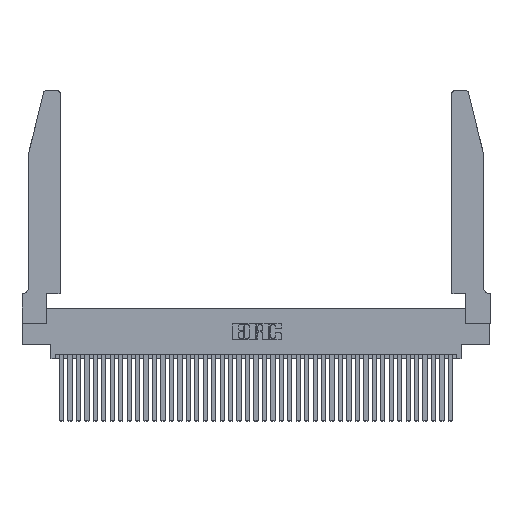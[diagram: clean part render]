
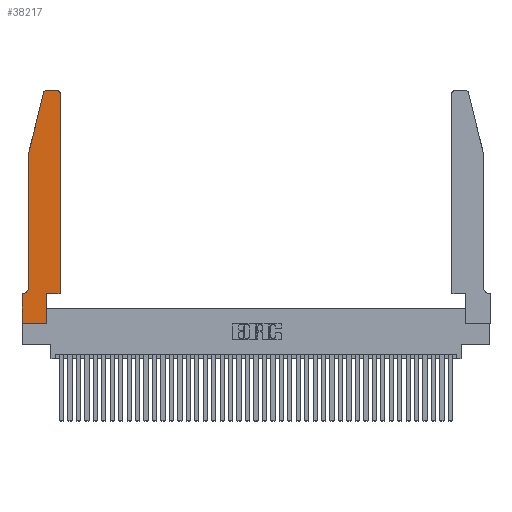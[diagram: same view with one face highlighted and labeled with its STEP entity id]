
A CAD part, top view. The second image highlights one B-rep face of the part: STEP entity #38217.
In plain terms, the highlighted planar face has unit normal (0, 0, 1).
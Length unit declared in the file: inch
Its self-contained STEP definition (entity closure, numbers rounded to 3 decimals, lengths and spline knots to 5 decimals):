
#286 = CARTESIAN_POINT ( 'NONE',  ( 0.0755, 2., 0.37 ) ) ;
#524 = ORIENTED_EDGE ( 'NONE', *, *, #22141, .T. ) ;
#861 = LINE ( 'NONE', #13321, #16793 ) ;
#1321 = DIRECTION ( 'NONE',  ( -1., 0., 0. ) ) ;
#1430 = VECTOR ( 'NONE', #27867, 39.37008 ) ;
#2955 = VECTOR ( 'NONE', #1321, 39.37008 ) ;
#3925 = AXIS2_PLACEMENT_3D ( 'NONE', #29279, #10418, #32471 ) ;
#3938 = LINE ( 'NONE', #17173, #2955 ) ;
#4411 = CARTESIAN_POINT ( 'NONE',  ( 0., 0.35, 0.37 ) ) ;
#4543 = VECTOR ( 'NONE', #5775, 39.37008 ) ;
#4550 = VERTEX_POINT ( 'NONE', #31764 ) ;
#4880 = CARTESIAN_POINT ( 'NONE',  ( 0.4205, 2.75, 0.37 ) ) ;
#5093 = ORIENTED_EDGE ( 'NONE', *, *, #18184, .T. ) ;
#5542 = CARTESIAN_POINT ( 'NONE',  ( 0.0755, 2., 0.37 ) ) ;
#5645 = EDGE_CURVE ( 'NONE', #4550, #9919, #6960, .T. ) ;
#5775 = DIRECTION ( 'NONE',  ( 0., -1., 0. ) ) ;
#6378 = VERTEX_POINT ( 'NONE', #24211 ) ;
#6424 = LINE ( 'NONE', #39726, #31275 ) ;
#6707 = CARTESIAN_POINT ( 'NONE',  ( 0.0055, 0.42, 0.37 ) ) ;
#6960 = LINE ( 'NONE', #31431, #38580 ) ;
#7142 = EDGE_CURVE ( 'NONE', #37734, #31909, #861, .T. ) ;
#7722 = EDGE_CURVE ( 'NONE', #31909, #20924, #31553, .T. ) ;
#7935 = VERTEX_POINT ( 'NONE', #23412 ) ;
#8237 = CARTESIAN_POINT ( 'NONE',  ( 0.2865, 0.35, 0.37 ) ) ;
#8771 = DIRECTION ( 'NONE',  ( 0., -1., 0. ) ) ;
#8877 = CARTESIAN_POINT ( 'NONE',  ( 0., 0., 0.37 ) ) ;
#9084 = EDGE_CURVE ( 'NONE', #11358, #6378, #14063, .T. ) ;
#9573 = LINE ( 'NONE', #5542, #25326 ) ;
#9919 = VERTEX_POINT ( 'NONE', #286 ) ;
#9966 = DIRECTION ( 'NONE',  ( -1., 0., 0. ) ) ;
#10418 = DIRECTION ( 'NONE',  ( 0., 0., 1. ) ) ;
#10712 = DIRECTION ( 'NONE',  ( 0., 0., 1. ) ) ;
#10796 = VERTEX_POINT ( 'NONE', #14861 ) ;
#10889 = DIRECTION ( 'NONE',  ( 1., 0., 0. ) ) ;
#11332 = DIRECTION ( 'NONE',  ( 0., 1., 0. ) ) ;
#11358 = VERTEX_POINT ( 'NONE', #38369 ) ;
#11906 = VERTEX_POINT ( 'NONE', #34550 ) ;
#13321 = CARTESIAN_POINT ( 'NONE',  ( 0.4505, 0.35, 0.37 ) ) ;
#13473 = CIRCLE ( 'NONE', #3925, 0.03 ) ;
#13902 = ORIENTED_EDGE ( 'NONE', *, *, #18046, .T. ) ;
#14063 = LINE ( 'NONE', #8877, #4543 ) ;
#14861 = CARTESIAN_POINT ( 'NONE',  ( 0.2865, 0., 0.37 ) ) ;
#15097 = FACE_OUTER_BOUND ( 'NONE', #16533, .T. ) ;
#15111 = ORIENTED_EDGE ( 'NONE', *, *, #9084, .T. ) ;
#16533 = EDGE_LOOP ( 'NONE', ( #13902, #18763, #20365, #34721, #16781, #524, #15111, #5093, #27080, #22132, #33124, #27763 ) ) ;
#16781 = ORIENTED_EDGE ( 'NONE', *, *, #16852, .T. ) ;
#16793 = VECTOR ( 'NONE', #38467, 39.37008 ) ;
#16852 = EDGE_CURVE ( 'NONE', #7935, #11906, #24384, .T. ) ;
#17173 = CARTESIAN_POINT ( 'NONE',  ( 0.2605, 2.75, 0.37 ) ) ;
#18046 = EDGE_CURVE ( 'NONE', #37634, #21155, #3938, .T. ) ;
#18184 = EDGE_CURVE ( 'NONE', #6378, #10796, #6424, .T. ) ;
#18384 = CARTESIAN_POINT ( 'NONE',  ( 0.0755, 0.35, 0.37 ) ) ;
#18731 = DIRECTION ( 'NONE',  ( -0.239, -0.971, 0. ) ) ;
#18736 = AXIS2_PLACEMENT_3D ( 'NONE', #29575, #10712, #32776 ) ;
#18763 = ORIENTED_EDGE ( 'NONE', *, *, #21801, .T. ) ;
#20365 = ORIENTED_EDGE ( 'NONE', *, *, #5645, .T. ) ;
#20545 = AXIS2_PLACEMENT_3D ( 'NONE', #4411, #29741, #10889 ) ;
#20924 = VERTEX_POINT ( 'NONE', #40758 ) ;
#21155 = VERTEX_POINT ( 'NONE', #29339 ) ;
#21801 = EDGE_CURVE ( 'NONE', #21155, #4550, #13473, .T. ) ;
#21918 = LINE ( 'NONE', #8237, #29298 ) ;
#22132 = ORIENTED_EDGE ( 'NONE', *, *, #7142, .T. ) ;
#22141 = EDGE_CURVE ( 'NONE', #11906, #11358, #25676, .T. ) ;
#23149 = VECTOR ( 'NONE', #35043, 39.37008 ) ;
#23412 = CARTESIAN_POINT ( 'NONE',  ( 0.0755, 0.42, 0.37 ) ) ;
#24211 = CARTESIAN_POINT ( 'NONE',  ( 0., 0., 0.37 ) ) ;
#24384 = CIRCLE ( 'NONE', #28872, 0.07 ) ;
#25326 = VECTOR ( 'NONE', #8771, 39.37008 ) ;
#25456 = CARTESIAN_POINT ( 'NONE',  ( 0.4505, 0.35, 0.37 ) ) ;
#25676 = LINE ( 'NONE', #18384, #1430 ) ;
#26019 = CARTESIAN_POINT ( 'NONE',  ( 0.4505, 0.35, 0.37 ) ) ;
#26534 = PLANE ( 'NONE',  #20545 ) ;
#27080 = ORIENTED_EDGE ( 'NONE', *, *, #32127, .T. ) ;
#27763 = ORIENTED_EDGE ( 'NONE', *, *, #40104, .T. ) ;
#27867 = DIRECTION ( 'NONE',  ( -1., 0., 0. ) ) ;
#28831 = DIRECTION ( 'NONE',  ( 0., 0., -1. ) ) ;
#28872 = AXIS2_PLACEMENT_3D ( 'NONE', #6707, #28831, #9966 ) ;
#29279 = CARTESIAN_POINT ( 'NONE',  ( 0.284, 2.72, 0.37 ) ) ;
#29298 = VECTOR ( 'NONE', #11332, 39.37008 ) ;
#29339 = CARTESIAN_POINT ( 'NONE',  ( 0.284, 2.75, 0.37 ) ) ;
#29575 = CARTESIAN_POINT ( 'NONE',  ( 0.4205, 2.72, 0.37 ) ) ;
#29741 = DIRECTION ( 'NONE',  ( 0., 0., 1. ) ) ;
#30398 = DIRECTION ( 'NONE',  ( 1., 0., 0. ) ) ;
#30763 = CARTESIAN_POINT ( 'NONE',  ( 0.2865, 0.35, 0.37 ) ) ;
#31275 = VECTOR ( 'NONE', #30398, 39.37008 ) ;
#31431 = CARTESIAN_POINT ( 'NONE',  ( 0.0755, 2., 0.37 ) ) ;
#31553 = LINE ( 'NONE', #25456, #23149 ) ;
#31764 = CARTESIAN_POINT ( 'NONE',  ( 0.25487, 2.72718, 0.37 ) ) ;
#31909 = VERTEX_POINT ( 'NONE', #26019 ) ;
#32127 = EDGE_CURVE ( 'NONE', #10796, #37734, #21918, .T. ) ;
#32471 = DIRECTION ( 'NONE',  ( 1., 0., 0. ) ) ;
#32776 = DIRECTION ( 'NONE',  ( 1., 0., 0. ) ) ;
#33124 = ORIENTED_EDGE ( 'NONE', *, *, #7722, .T. ) ;
#34550 = CARTESIAN_POINT ( 'NONE',  ( 0.0055, 0.35, 0.37 ) ) ;
#34721 = ORIENTED_EDGE ( 'NONE', *, *, #39687, .T. ) ;
#34735 = CIRCLE ( 'NONE', #18736, 0.03 ) ;
#35043 = DIRECTION ( 'NONE',  ( 0., 1., 0. ) ) ;
#37634 = VERTEX_POINT ( 'NONE', #4880 ) ;
#37734 = VERTEX_POINT ( 'NONE', #30763 ) ;
#38217 = ADVANCED_FACE ( 'NONE', ( #15097 ), #26534, .T. ) ;
#38369 = CARTESIAN_POINT ( 'NONE',  ( 0., 0.35, 0.37 ) ) ;
#38467 = DIRECTION ( 'NONE',  ( 1., 0., 0. ) ) ;
#38580 = VECTOR ( 'NONE', #18731, 39.37008 ) ;
#39687 = EDGE_CURVE ( 'NONE', #9919, #7935, #9573, .T. ) ;
#39726 = CARTESIAN_POINT ( 'NONE',  ( 0., 0., 0.37 ) ) ;
#40104 = EDGE_CURVE ( 'NONE', #20924, #37634, #34735, .T. ) ;
#40758 = CARTESIAN_POINT ( 'NONE',  ( 0.4505, 2.72, 0.37 ) ) ;
